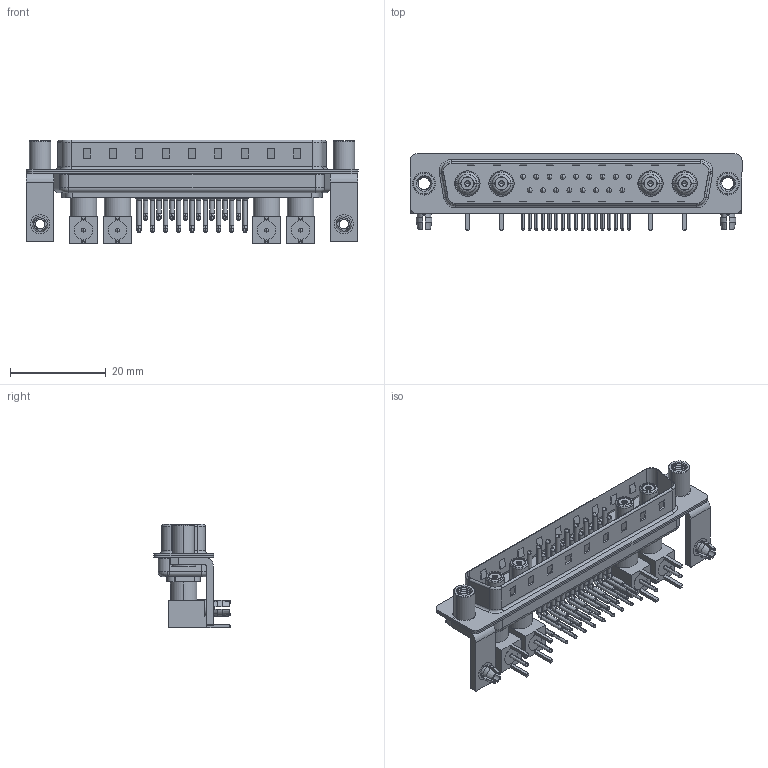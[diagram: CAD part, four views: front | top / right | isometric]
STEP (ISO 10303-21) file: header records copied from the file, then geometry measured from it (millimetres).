
FILE_DESCRIPTION (( 'STEP AP203' ), '1' );
FILE_NAME ('629-21W4640-7TD.STEP', '2022-05-17T08:10:34', ( '' ), ( '' ), 'SwSTEP 2.0', 'SolidWorks 2020', '' );
FILE_SCHEMA (( 'CONFIG_CONTROL_DESIGN' ));
Length unit declared in the file: millimetre
Products named in the file (20): Co-Ax Jack Assy_RA; Insulator Socket 2; 629Combo Contact Row 2; Insulator RA Pin; Socket_RA; Co-Ax Jack_RA PC Tail; 629Combo Shell Rear_37 Contacts; RA Back Shell; 629Combo Shell Front_37 Contacts; 629Combo Stabilizer Bracket; 629Combo Contact Row 1; 629Combo Threaded Standoff_D; Locking Collar; 629Combo Board Lock; Insulator Socket; 629-21W4640-7TD; 629Combo Housing_21W4
Assembly tree (58 placements, depth 3):
  629-21W4640-7TD
    629Combo Housing_21W4
    629Combo Shell Rear_37 Contacts
    629Combo Shell Front_37 Contacts
    629Combo Stabilizer Bracket  x2
    629Combo Board Lock  x2
    629Combo Threaded Standoff_D  x2
    Co-Ax Jack Assy_RA
      Co-Ax Jack_RA PC Tail
      Insulator Socket
      Insulator Socket 2
      Locking Collar
      Socket_RA
      RA Back Shell
      Insulator RA Pin
    Co-Ax Jack Assy_RA
      Co-Ax Jack_RA PC Tail
      Insulator Socket
      Insulator Socket 2
      Locking Collar
      Socket_RA
      RA Back Shell
      Insulator RA Pin
    Co-Ax Jack Assy_RA
      Co-Ax Jack_RA PC Tail
      Insulator Socket
      Insulator Socket 2
      Locking Collar
      Socket_RA
      RA Back Shell
      Insulator RA Pin
    Co-Ax Jack Assy_RA
      Co-Ax Jack_RA PC Tail
      Insulator Socket
      Insulator Socket 2
      Locking Collar
      Socket_RA
      RA Back Shell
      Insulator RA Pin
    629Combo Contact Row 1  x9
    629Combo Contact Row 2  x8
Bounding box: 69.4 x 16 x 21.71 mm (x, y, z)
Volume: 5468.3 mm3; surface area: 14621.2 mm2
Topology: 54 solids, 54 shells, 3080 faces, 8239 edges, 5308 vertices
Faces by surface type: plane 1589, cylinder 1125, cone 172, bspline 112, torus 74, sphere 8
Entity records: 35669 total; most frequent: CARTESIAN_POINT 7951, DIRECTION 5348, ORIENTED_EDGE 4972, EDGE_CURVE 2486, AXIS2_PLACEMENT_3D 1948, VERTEX_POINT 1604, VECTOR 1452, LINE 1452
